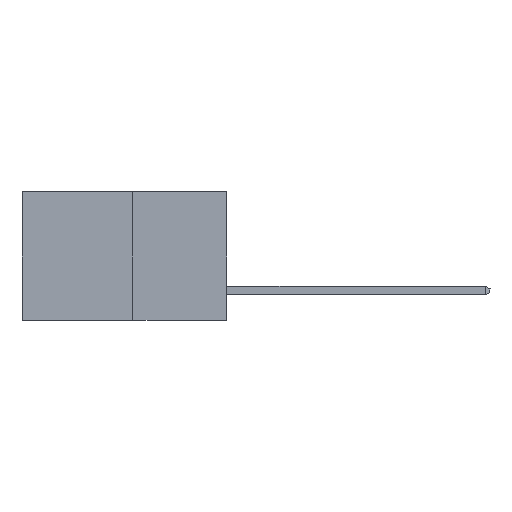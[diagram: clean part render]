
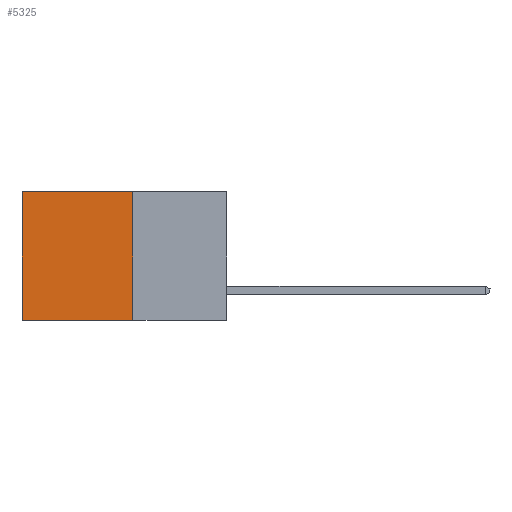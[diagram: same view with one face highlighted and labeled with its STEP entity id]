
A CAD part, left-side view. The second image highlights one B-rep face of the part: STEP entity #5325.
In plain terms, the highlighted planar face has unit normal (-1, 0, 0).
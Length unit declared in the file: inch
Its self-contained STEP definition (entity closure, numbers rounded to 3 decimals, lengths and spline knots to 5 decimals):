
#600 = CARTESIAN_POINT ( 'NONE',  ( 0.277, 0.27, -0.37 ) ) ;
#1827 = CARTESIAN_POINT ( 'NONE',  ( 0.277, 0.27, 0. ) ) ;
#1949 = VERTEX_POINT ( 'NONE', #1827 ) ;
#2217 = EDGE_CURVE ( 'NONE', #1949, #13427, #11290, .T. ) ;
#2803 = CARTESIAN_POINT ( 'NONE',  ( 0.277, 0.27, 0. ) ) ;
#3263 = EDGE_CURVE ( 'NONE', #10439, #12863, #3736, .T. ) ;
#3736 = LINE ( 'NONE', #9506, #10827 ) ;
#3741 = EDGE_CURVE ( 'NONE', #1949, #10439, #16825, .T. ) ;
#4289 = EDGE_LOOP ( 'NONE', ( #7049, #7172, #7487, #7550 ) ) ;
#5325 = ADVANCED_FACE ( 'NONE', ( #15977 ), #13200, .F. ) ;
#6493 = DIRECTION ( 'NONE',  ( 0., 1., 0. ) ) ;
#6568 = AXIS2_PLACEMENT_3D ( 'NONE', #13337, #13197, #13174 ) ;
#7049 = ORIENTED_EDGE ( 'NONE', *, *, #11418, .T. ) ;
#7172 = ORIENTED_EDGE ( 'NONE', *, *, #3263, .F. ) ;
#7487 = ORIENTED_EDGE ( 'NONE', *, *, #3741, .F. ) ;
#7550 = ORIENTED_EDGE ( 'NONE', *, *, #2217, .T. ) ;
#7762 = CARTESIAN_POINT ( 'NONE',  ( 0.277, 0.59, -0.37 ) ) ;
#7923 = DIRECTION ( 'NONE',  ( 0., 0., -1. ) ) ;
#8352 = DIRECTION ( 'NONE',  ( 0., 0., -1. ) ) ;
#8394 = CARTESIAN_POINT ( 'NONE',  ( 0.277, 0.59, 0. ) ) ;
#8826 = VECTOR ( 'NONE', #7923, 39.37008 ) ;
#9506 = CARTESIAN_POINT ( 'NONE',  ( 0.277, 0.27, -0.37 ) ) ;
#9941 = CARTESIAN_POINT ( 'NONE',  ( 0.277, 0.27, -0.37 ) ) ;
#10439 = VERTEX_POINT ( 'NONE', #600 ) ;
#10827 = VECTOR ( 'NONE', #14720, 39.37008 ) ;
#11290 = LINE ( 'NONE', #2803, #17470 ) ;
#11418 = EDGE_CURVE ( 'NONE', #13427, #12863, #15584, .T. ) ;
#12863 = VERTEX_POINT ( 'NONE', #16810 ) ;
#13174 = DIRECTION ( 'NONE',  ( 0., 0., -1. ) ) ;
#13197 = DIRECTION ( 'NONE',  ( 1., 0., 0. ) ) ;
#13200 = PLANE ( 'NONE',  #6568 ) ;
#13337 = CARTESIAN_POINT ( 'NONE',  ( 0.277, 0.27, -0.37 ) ) ;
#13427 = VERTEX_POINT ( 'NONE', #8394 ) ;
#14720 = DIRECTION ( 'NONE',  ( 0., 1., 0. ) ) ;
#15584 = LINE ( 'NONE', #7762, #8826 ) ;
#15977 = FACE_OUTER_BOUND ( 'NONE', #4289, .T. ) ;
#16420 = VECTOR ( 'NONE', #8352, 39.37008 ) ;
#16810 = CARTESIAN_POINT ( 'NONE',  ( 0.277, 0.59, -0.37 ) ) ;
#16825 = LINE ( 'NONE', #9941, #16420 ) ;
#17470 = VECTOR ( 'NONE', #6493, 39.37008 ) ;
